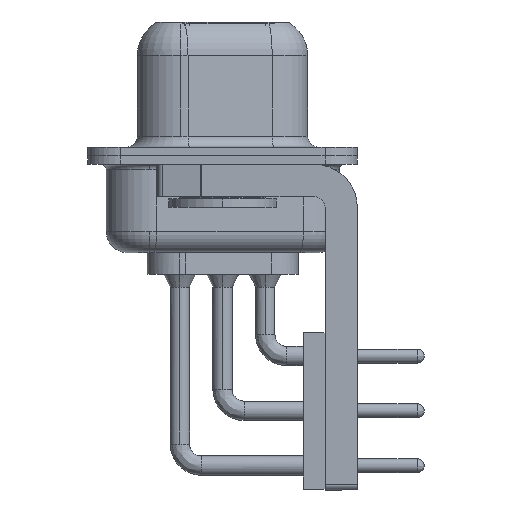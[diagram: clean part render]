
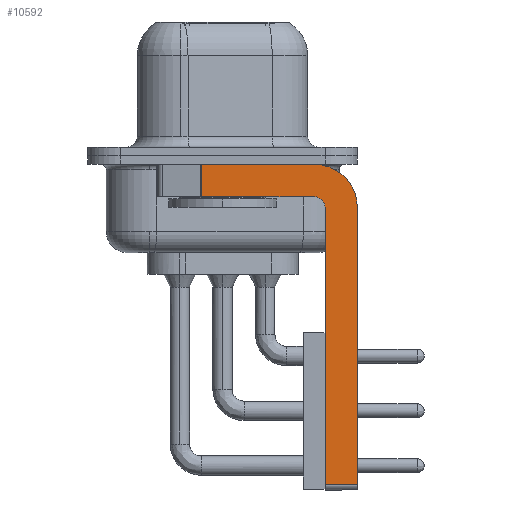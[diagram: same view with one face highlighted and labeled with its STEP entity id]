
A CAD part, left-side view. The second image highlights one B-rep face of the part: STEP entity #10592.
In plain terms, the highlighted planar face has unit normal (-1, 0, 0).
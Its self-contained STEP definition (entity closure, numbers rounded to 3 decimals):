
#165 = CARTESIAN_POINT ( 'NONE',  ( -2.9, -4.75, -2.4 ) ) ;
#586 = EDGE_CURVE ( 'NONE', #6441, #26508, #22355, .T. ) ;
#940 = VECTOR ( 'NONE', #8081, 1000. ) ;
#973 = VECTOR ( 'NONE', #25854, 1000. ) ;
#1133 = EDGE_CURVE ( 'NONE', #2191, #9598, #23669, .T. ) ;
#1201 = CARTESIAN_POINT ( 'NONE',  ( -2.9, 0.978, -1.9 ) ) ;
#1869 = DIRECTION ( 'NONE',  ( 0., 0., -1. ) ) ;
#2191 = VERTEX_POINT ( 'NONE', #11717 ) ;
#3012 = VERTEX_POINT ( 'NONE', #14545 ) ;
#3539 = EDGE_CURVE ( 'NONE', #2191, #4010, #15682, .T. ) ;
#4010 = VERTEX_POINT ( 'NONE', #4623 ) ;
#4018 = LINE ( 'NONE', #6371, #15658 ) ;
#4197 = EDGE_CURVE ( 'NONE', #6441, #3012, #4018, .T. ) ;
#4260 = ORIENTED_EDGE ( 'NONE', *, *, #15385, .F. ) ;
#4623 = CARTESIAN_POINT ( 'NONE',  ( -2.9, -6.25, -15.25 ) ) ;
#5532 = DIRECTION ( 'NONE',  ( -1., 0., 0. ) ) ;
#5948 = PLANE ( 'NONE',  #13101 ) ;
#6082 = AXIS2_PLACEMENT_3D ( 'NONE', #12074, #26639, #14161 ) ;
#6244 = DIRECTION ( 'NONE',  ( 0., -1., 0. ) ) ;
#6371 = CARTESIAN_POINT ( 'NONE',  ( -2.9, 3., -0.4 ) ) ;
#6441 = VERTEX_POINT ( 'NONE', #10362 ) ;
#6871 = EDGE_CURVE ( 'NONE', #3012, #22231, #21746, .T. ) ;
#7736 = VECTOR ( 'NONE', #24630, 1000. ) ;
#8026 = CARTESIAN_POINT ( 'NONE',  ( -2.9, -4.25, -2.4 ) ) ;
#8064 = ORIENTED_EDGE ( 'NONE', *, *, #6871, .F. ) ;
#8081 = DIRECTION ( 'NONE',  ( 0., 0., -1. ) ) ;
#8406 = ORIENTED_EDGE ( 'NONE', *, *, #3539, .T. ) ;
#9086 = CARTESIAN_POINT ( 'NONE',  ( -2.9, -6.25, -2.4 ) ) ;
#9170 = EDGE_LOOP ( 'NONE', ( #15721, #18635, #20930, #11317, #19265, #8406, #4260, #8064 ) ) ;
#9598 = VERTEX_POINT ( 'NONE', #165 ) ;
#10174 = VECTOR ( 'NONE', #26600, 1000. ) ;
#10362 = CARTESIAN_POINT ( 'NONE',  ( -2.9, 0.978, -0.4 ) ) ;
#10441 = EDGE_CURVE ( 'NONE', #9598, #17355, #12138, .T. ) ;
#10592 = ADVANCED_FACE ( 'NONE', ( #24832 ), #5948, .F. ) ;
#11279 = LINE ( 'NONE', #22591, #940 ) ;
#11317 = ORIENTED_EDGE ( 'NONE', *, *, #10441, .F. ) ;
#11717 = CARTESIAN_POINT ( 'NONE',  ( -2.9, -4.75, -15.25 ) ) ;
#12074 = CARTESIAN_POINT ( 'NONE',  ( -2.9, -4.25, -2.4 ) ) ;
#12138 = CIRCLE ( 'NONE', #17776, 0.5 ) ;
#12289 = CARTESIAN_POINT ( 'NONE',  ( -2.9, -4.25, -1.9 ) ) ;
#13101 = AXIS2_PLACEMENT_3D ( 'NONE', #8026, #14272, #1869 ) ;
#14161 = DIRECTION ( 'NONE',  ( 0., 0., -1. ) ) ;
#14272 = DIRECTION ( 'NONE',  ( 1., 0., 0. ) ) ;
#14545 = CARTESIAN_POINT ( 'NONE',  ( -2.9, -4.25, -0.4 ) ) ;
#15385 = EDGE_CURVE ( 'NONE', #22231, #4010, #11279, .T. ) ;
#15658 = VECTOR ( 'NONE', #6244, 1000. ) ;
#15682 = LINE ( 'NONE', #25712, #10174 ) ;
#15721 = ORIENTED_EDGE ( 'NONE', *, *, #4197, .F. ) ;
#16966 = CARTESIAN_POINT ( 'NONE',  ( -2.9, 0.978, -1.9 ) ) ;
#17355 = VERTEX_POINT ( 'NONE', #24583 ) ;
#17776 = AXIS2_PLACEMENT_3D ( 'NONE', #17914, #5532, #20001 ) ;
#17914 = CARTESIAN_POINT ( 'NONE',  ( -2.9, -4.25, -2.4 ) ) ;
#18635 = ORIENTED_EDGE ( 'NONE', *, *, #586, .T. ) ;
#19265 = ORIENTED_EDGE ( 'NONE', *, *, #1133, .F. ) ;
#20001 = DIRECTION ( 'NONE',  ( 0., 0., 1. ) ) ;
#20930 = ORIENTED_EDGE ( 'NONE', *, *, #21321, .F. ) ;
#21321 = EDGE_CURVE ( 'NONE', #17355, #26508, #25037, .T. ) ;
#21746 = CIRCLE ( 'NONE', #6082, 2. ) ;
#22231 = VERTEX_POINT ( 'NONE', #9086 ) ;
#22355 = LINE ( 'NONE', #16966, #973 ) ;
#22591 = CARTESIAN_POINT ( 'NONE',  ( -2.9, -6.25, -2.4 ) ) ;
#23669 = LINE ( 'NONE', #24873, #7736 ) ;
#24391 = VECTOR ( 'NONE', #24751, 1000. ) ;
#24583 = CARTESIAN_POINT ( 'NONE',  ( -2.9, -4.25, -1.9 ) ) ;
#24630 = DIRECTION ( 'NONE',  ( 0., 0., 1. ) ) ;
#24751 = DIRECTION ( 'NONE',  ( 0., 1., 0. ) ) ;
#24832 = FACE_OUTER_BOUND ( 'NONE', #9170, .T. ) ;
#24873 = CARTESIAN_POINT ( 'NONE',  ( -2.9, -4.75, -15.5 ) ) ;
#25037 = LINE ( 'NONE', #12289, #24391 ) ;
#25712 = CARTESIAN_POINT ( 'NONE',  ( -2.9, -4.25, -15.25 ) ) ;
#25854 = DIRECTION ( 'NONE',  ( 0., 0., -1. ) ) ;
#26508 = VERTEX_POINT ( 'NONE', #1201 ) ;
#26600 = DIRECTION ( 'NONE',  ( 0., -1., 0. ) ) ;
#26639 = DIRECTION ( 'NONE',  ( 1., 0., 0. ) ) ;
